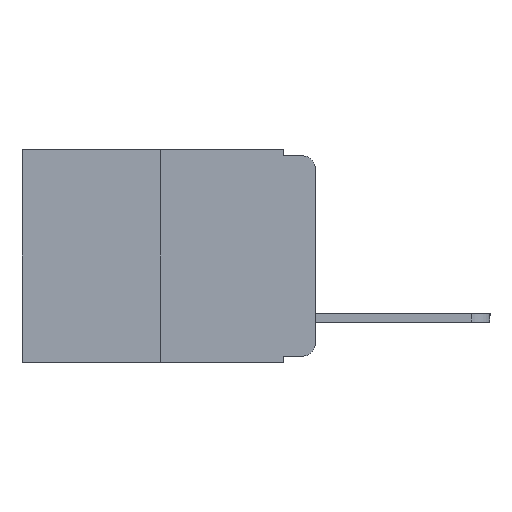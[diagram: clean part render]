
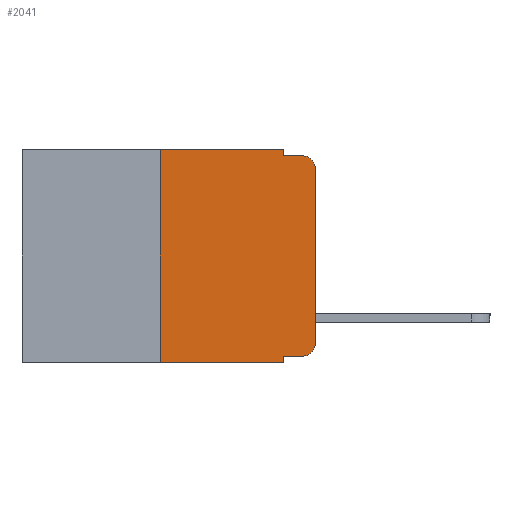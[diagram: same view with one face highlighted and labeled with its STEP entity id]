
A CAD part, left-side view. The second image highlights one B-rep face of the part: STEP entity #2041.
In plain terms, the highlighted planar face has unit normal (-1, 0, 0).
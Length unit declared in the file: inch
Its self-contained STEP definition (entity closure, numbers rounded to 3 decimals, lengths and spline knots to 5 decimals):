
#97 = ORIENTED_EDGE ( 'NONE', *, *, #6870, .F. ) ;
#128 = EDGE_CURVE ( 'NONE', #11298, #6250, #6833, .T. ) ;
#283 = VERTEX_POINT ( 'NONE', #4449 ) ;
#416 = EDGE_CURVE ( 'NONE', #550, #2827, #8573, .T. ) ;
#550 = VERTEX_POINT ( 'NONE', #7133 ) ;
#833 = EDGE_CURVE ( 'NONE', #2375, #11298, #8929, .T. ) ;
#982 = VECTOR ( 'NONE', #7515, 39.37008 ) ;
#1508 = CARTESIAN_POINT ( 'NONE',  ( 0., 0.02, -0.333 ) ) ;
#1691 = DIRECTION ( 'NONE',  ( -1., 0., 0. ) ) ;
#1694 = CARTESIAN_POINT ( 'NONE',  ( 0., 0.02, -0.313 ) ) ;
#1706 = DIRECTION ( 'NONE',  ( 0., 0., -1. ) ) ;
#1958 = VECTOR ( 'NONE', #8896, 39.37008 ) ;
#1961 = VECTOR ( 'NONE', #9147, 39.37008 ) ;
#2041 = ADVANCED_FACE ( 'NONE', ( #3944 ), #2843, .F. ) ;
#2254 = ORIENTED_EDGE ( 'NONE', *, *, #8599, .F. ) ;
#2375 = VERTEX_POINT ( 'NONE', #4605 ) ;
#2706 = AXIS2_PLACEMENT_3D ( 'NONE', #1694, #1691, #1706 ) ;
#2827 = VERTEX_POINT ( 'NONE', #9362 ) ;
#2843 = PLANE ( 'NONE',  #10447 ) ;
#2896 = ORIENTED_EDGE ( 'NONE', *, *, #6268, .T. ) ;
#3785 = LINE ( 'NONE', #9375, #10465 ) ;
#3828 = CARTESIAN_POINT ( 'NONE',  ( 0., 0.473, 0. ) ) ;
#3830 = DIRECTION ( 'NONE',  ( 0., -1., 0. ) ) ;
#3936 = CARTESIAN_POINT ( 'NONE',  ( 0., 0.02, -0.01 ) ) ;
#3940 = ORIENTED_EDGE ( 'NONE', *, *, #11347, .F. ) ;
#3944 = FACE_OUTER_BOUND ( 'NONE', #5223, .T. ) ;
#3984 = VECTOR ( 'NONE', #3830, 39.37008 ) ;
#4006 = CIRCLE ( 'NONE', #2706, 0.02 ) ;
#4113 = LINE ( 'NONE', #10755, #6251 ) ;
#4253 = LINE ( 'NONE', #8067, #1958 ) ;
#4449 = CARTESIAN_POINT ( 'NONE',  ( 0., 0.25, -0.343 ) ) ;
#4605 = CARTESIAN_POINT ( 'NONE',  ( 0., 0., -0.313 ) ) ;
#4777 = AXIS2_PLACEMENT_3D ( 'NONE', #9171, #9191, #9080 ) ;
#4813 = CARTESIAN_POINT ( 'NONE',  ( 0., 0.051, 0. ) ) ;
#5223 = EDGE_LOOP ( 'NONE', ( #9943, #8262, #3940, #8916, #11109, #2254, #11616, #97, #2896, #7750 ) ) ;
#5382 = DIRECTION ( 'NONE',  ( 0., -1., 0. ) ) ;
#5676 = EDGE_CURVE ( 'NONE', #11289, #2375, #4006, .T. ) ;
#5774 = DIRECTION ( 'NONE',  ( 1., 0., 0. ) ) ;
#5982 = DIRECTION ( 'NONE',  ( 0., 0., -1. ) ) ;
#6250 = VERTEX_POINT ( 'NONE', #3936 ) ;
#6251 = VECTOR ( 'NONE', #6548, 39.37008 ) ;
#6268 = EDGE_CURVE ( 'NONE', #11456, #11289, #10901, .T. ) ;
#6392 = LINE ( 'NONE', #9913, #3984 ) ;
#6452 = CARTESIAN_POINT ( 'NONE',  ( 0., 0.473, 0. ) ) ;
#6548 = DIRECTION ( 'NONE',  ( 0., 0., 1. ) ) ;
#6802 = EDGE_CURVE ( 'NONE', #283, #10971, #6392, .T. ) ;
#6833 = CIRCLE ( 'NONE', #4777, 0.02 ) ;
#6870 = EDGE_CURVE ( 'NONE', #11456, #10971, #11142, .T. ) ;
#7133 = CARTESIAN_POINT ( 'NONE',  ( 0., 0.25, 0. ) ) ;
#7515 = DIRECTION ( 'NONE',  ( 0., 0., -1. ) ) ;
#7750 = ORIENTED_EDGE ( 'NONE', *, *, #5676, .T. ) ;
#7965 = CARTESIAN_POINT ( 'NONE',  ( 0., 0.051, -0.01 ) ) ;
#8067 = CARTESIAN_POINT ( 'NONE',  ( 0., 0.051, -0.01 ) ) ;
#8172 = CARTESIAN_POINT ( 'NONE',  ( 0., 0.051, -0.333 ) ) ;
#8246 = CARTESIAN_POINT ( 'NONE',  ( 0., 0.051, -0.333 ) ) ;
#8262 = ORIENTED_EDGE ( 'NONE', *, *, #128, .T. ) ;
#8540 = DIRECTION ( 'NONE',  ( 0., 0., -1. ) ) ;
#8573 = LINE ( 'NONE', #3828, #10759 ) ;
#8599 = EDGE_CURVE ( 'NONE', #283, #550, #4113, .T. ) ;
#8896 = DIRECTION ( 'NONE',  ( 0., -1., 0. ) ) ;
#8916 = ORIENTED_EDGE ( 'NONE', *, *, #9709, .F. ) ;
#8929 = LINE ( 'NONE', #9193, #1961 ) ;
#9080 = DIRECTION ( 'NONE',  ( 0., 0., -1. ) ) ;
#9147 = DIRECTION ( 'NONE',  ( 0., 0., 1. ) ) ;
#9171 = CARTESIAN_POINT ( 'NONE',  ( 0., 0.02, -0.03 ) ) ;
#9191 = DIRECTION ( 'NONE',  ( -1., 0., 0. ) ) ;
#9193 = CARTESIAN_POINT ( 'NONE',  ( 0., 0., 0. ) ) ;
#9308 = CARTESIAN_POINT ( 'NONE',  ( 0., 0.051, -0.343 ) ) ;
#9362 = CARTESIAN_POINT ( 'NONE',  ( 0., 0.051, 0. ) ) ;
#9375 = CARTESIAN_POINT ( 'NONE',  ( 0., 0.051, 0. ) ) ;
#9701 = CARTESIAN_POINT ( 'NONE',  ( 0., 0., -0.03 ) ) ;
#9709 = EDGE_CURVE ( 'NONE', #2827, #11236, #3785, .T. ) ;
#9913 = CARTESIAN_POINT ( 'NONE',  ( 0., 0.473, -0.343 ) ) ;
#9943 = ORIENTED_EDGE ( 'NONE', *, *, #833, .T. ) ;
#10447 = AXIS2_PLACEMENT_3D ( 'NONE', #6452, #5774, #5982 ) ;
#10465 = VECTOR ( 'NONE', #8540, 39.37008 ) ;
#10502 = DIRECTION ( 'NONE',  ( 0., -1., 0. ) ) ;
#10643 = VECTOR ( 'NONE', #10502, 39.37008 ) ;
#10755 = CARTESIAN_POINT ( 'NONE',  ( 0., 0.25, 0. ) ) ;
#10759 = VECTOR ( 'NONE', #5382, 39.37008 ) ;
#10901 = LINE ( 'NONE', #8246, #10643 ) ;
#10971 = VERTEX_POINT ( 'NONE', #9308 ) ;
#11109 = ORIENTED_EDGE ( 'NONE', *, *, #416, .F. ) ;
#11142 = LINE ( 'NONE', #4813, #982 ) ;
#11236 = VERTEX_POINT ( 'NONE', #7965 ) ;
#11289 = VERTEX_POINT ( 'NONE', #1508 ) ;
#11298 = VERTEX_POINT ( 'NONE', #9701 ) ;
#11347 = EDGE_CURVE ( 'NONE', #11236, #6250, #4253, .T. ) ;
#11456 = VERTEX_POINT ( 'NONE', #8172 ) ;
#11616 = ORIENTED_EDGE ( 'NONE', *, *, #6802, .T. ) ;
